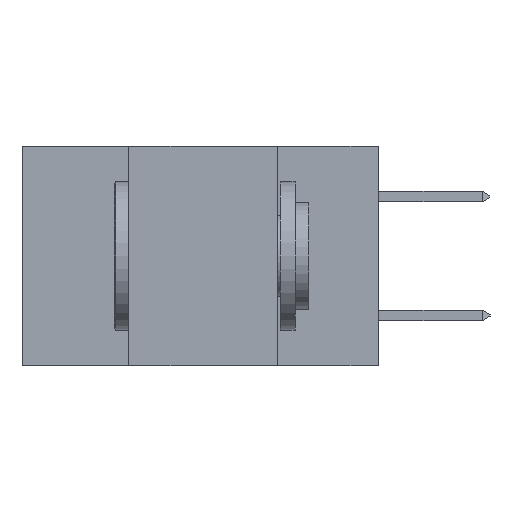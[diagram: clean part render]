
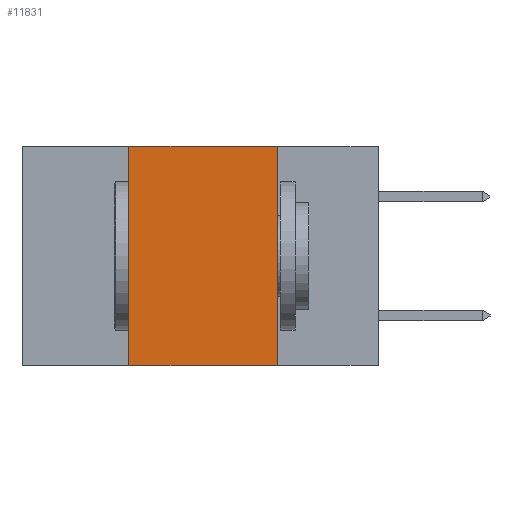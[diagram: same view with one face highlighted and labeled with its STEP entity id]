
A CAD part, left-side view. The second image highlights one B-rep face of the part: STEP entity #11831.
In plain terms, the highlighted planar face has unit normal (-1, 0, 0).
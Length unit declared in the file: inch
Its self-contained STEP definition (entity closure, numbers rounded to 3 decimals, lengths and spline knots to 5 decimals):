
#1071 = CARTESIAN_POINT ( 'NONE',  ( 0., 0.6, 0. ) ) ;
#1640 = LINE ( 'NONE', #7426, #6157 ) ;
#1765 = DIRECTION ( 'NONE',  ( 0., 0., -1. ) ) ;
#3278 = CARTESIAN_POINT ( 'NONE',  ( 0., 0.17, 0. ) ) ;
#4397 = CARTESIAN_POINT ( 'NONE',  ( 0., 0.6, -0.37 ) ) ;
#4572 = DIRECTION ( 'NONE',  ( 0., -1., 0. ) ) ;
#5339 = ORIENTED_EDGE ( 'NONE', *, *, #15623, .F. ) ;
#5600 = EDGE_CURVE ( 'NONE', #13795, #20683, #15495, .T. ) ;
#6157 = VECTOR ( 'NONE', #19200, 39.37008 ) ;
#6957 = LINE ( 'NONE', #1071, #19821 ) ;
#6996 = EDGE_CURVE ( 'NONE', #10028, #16907, #6957, .T. ) ;
#7426 = CARTESIAN_POINT ( 'NONE',  ( 0., 0.42, -0.37 ) ) ;
#7530 = DIRECTION ( 'NONE',  ( 1., 0., 0. ) ) ;
#7658 = CARTESIAN_POINT ( 'NONE',  ( 0., 0.17, -0.37 ) ) ;
#8201 = LINE ( 'NONE', #15324, #11097 ) ;
#9117 = CARTESIAN_POINT ( 'NONE',  ( 0., 0.42, -0.37 ) ) ;
#10028 = VERTEX_POINT ( 'NONE', #11504 ) ;
#10979 = VECTOR ( 'NONE', #4572, 39.37008 ) ;
#11097 = VECTOR ( 'NONE', #1765, 39.37008 ) ;
#11504 = CARTESIAN_POINT ( 'NONE',  ( 0., 0.42, 0. ) ) ;
#11831 = ADVANCED_FACE ( 'NONE', ( #12553 ), #12548, .F. ) ;
#12548 = PLANE ( 'NONE',  #15954 ) ;
#12553 = FACE_OUTER_BOUND ( 'NONE', #20988, .T. ) ;
#13786 = EDGE_CURVE ( 'NONE', #13795, #10028, #1640, .T. ) ;
#13795 = VERTEX_POINT ( 'NONE', #9117 ) ;
#14269 = CARTESIAN_POINT ( 'NONE',  ( 0., 0.6, 0. ) ) ;
#14661 = DIRECTION ( 'NONE',  ( 0., -1., 0. ) ) ;
#15324 = CARTESIAN_POINT ( 'NONE',  ( 0., 0.17, -0.37 ) ) ;
#15495 = LINE ( 'NONE', #4397, #10979 ) ;
#15623 = EDGE_CURVE ( 'NONE', #16907, #20683, #8201, .T. ) ;
#15954 = AXIS2_PLACEMENT_3D ( 'NONE', #14269, #7530, #19291 ) ;
#16722 = ORIENTED_EDGE ( 'NONE', *, *, #13786, .F. ) ;
#16907 = VERTEX_POINT ( 'NONE', #3278 ) ;
#17259 = ORIENTED_EDGE ( 'NONE', *, *, #6996, .F. ) ;
#18272 = ORIENTED_EDGE ( 'NONE', *, *, #5600, .T. ) ;
#19200 = DIRECTION ( 'NONE',  ( 0., 0., 1. ) ) ;
#19291 = DIRECTION ( 'NONE',  ( 0., 0., -1. ) ) ;
#19821 = VECTOR ( 'NONE', #14661, 39.37008 ) ;
#20683 = VERTEX_POINT ( 'NONE', #7658 ) ;
#20988 = EDGE_LOOP ( 'NONE', ( #5339, #17259, #16722, #18272 ) ) ;
